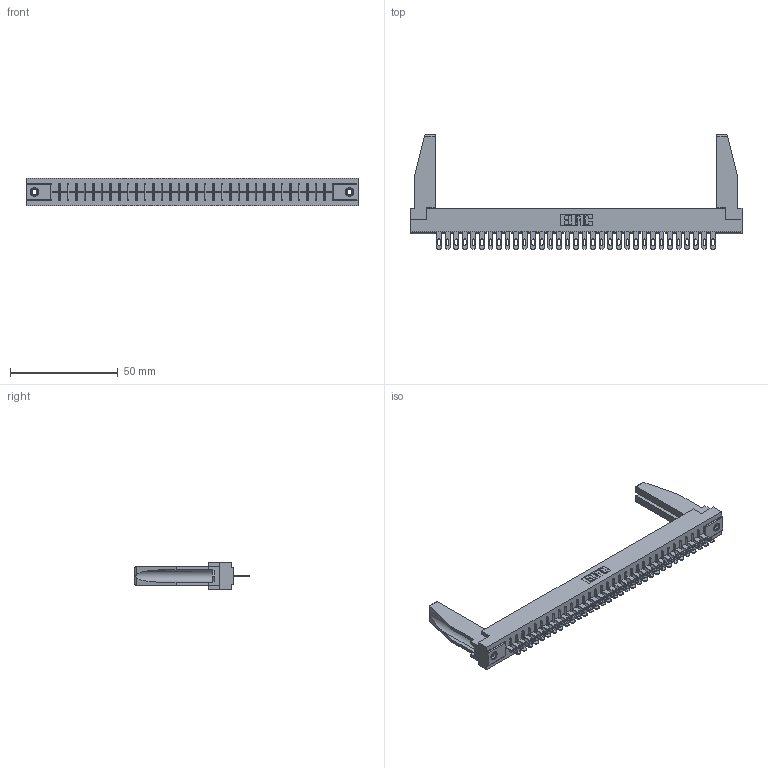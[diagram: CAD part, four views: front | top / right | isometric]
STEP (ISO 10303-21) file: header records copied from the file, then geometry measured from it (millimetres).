
FILE_DESCRIPTION (( 'STEP AP203' ), '1' );
FILE_NAME ('316-033-400-178.STEP', '2020-09-23T02:03:36', ( '' ), ( '' ), 'SwSTEP 2.0', 'SolidWorks 2020', '' );
FILE_SCHEMA (( 'CONFIG_CONTROL_DESIGN' ));
Length unit declared in the file: inch
Products named in the file (5): 345-250-001_345-250-001-102; 306 Part_.156 Dia; 316-033-400-178; 307-220-078; 306-290-001_100
Assembly tree (38 placements, depth 2):
  316-033-400-178
    306 Part_.156 Dia
    306-290-001_100  x33
    345-250-001_345-250-001-102  x2
    307-220-078  x2
Bounding box: 153.77 x 52.91 x 12.7 mm (x, y, z)
Volume: 21028.7 mm3; surface area: 21788.4 mm2
Topology: 38 solids, 38 shells, 2754 faces, 7741 edges, 4974 vertices
Faces by surface type: plane 1802, cylinder 804, sphere 132, cone 12, torus 4
Entity records: 34543 total; most frequent: CARTESIAN_POINT 5800, ORIENTED_EDGE 5708, DIRECTION 5672, EDGE_CURVE 2854, LINE 2228, VECTOR 2228, VERTEX_POINT 1808, AXIS2_PLACEMENT_3D 1722
